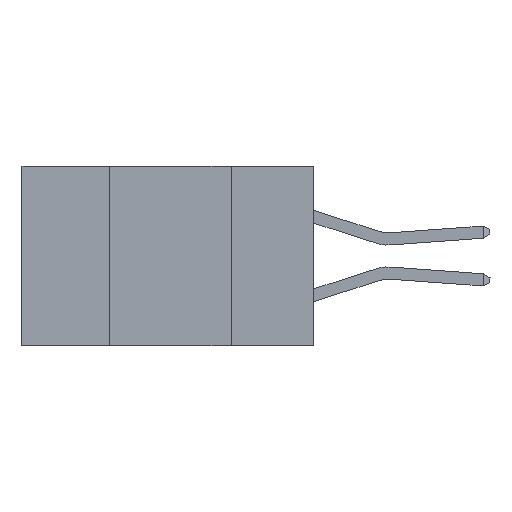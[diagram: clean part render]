
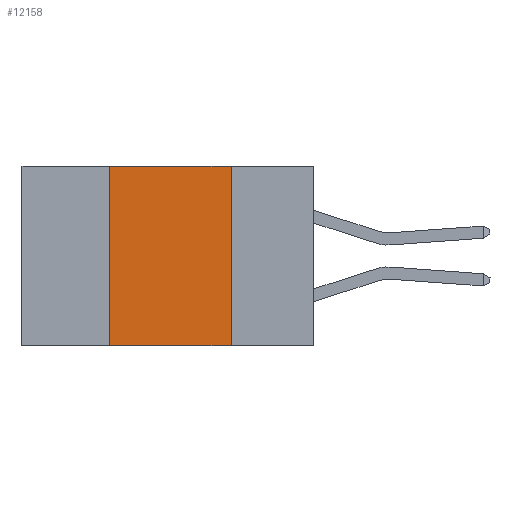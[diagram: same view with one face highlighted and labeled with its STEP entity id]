
A CAD part, left-side view. The second image highlights one B-rep face of the part: STEP entity #12158.
In plain terms, the highlighted planar face has unit normal (-1, 0, 0).
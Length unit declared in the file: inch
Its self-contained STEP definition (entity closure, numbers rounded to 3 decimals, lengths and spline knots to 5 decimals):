
#51 = EDGE_CURVE ( 'NONE', #9231, #17486, #16241, .T. ) ;
#1296 = ORIENTED_EDGE ( 'NONE', *, *, #18186, .F. ) ;
#1807 = VECTOR ( 'NONE', #5083, 39.37008 ) ;
#2206 = CARTESIAN_POINT ( 'NONE',  ( 0., 0.17, 0. ) ) ;
#2783 = DIRECTION ( 'NONE',  ( 0., 0., -1. ) ) ;
#3113 = VECTOR ( 'NONE', #12001, 39.37008 ) ;
#3127 = ORIENTED_EDGE ( 'NONE', *, *, #18317, .F. ) ;
#3414 = CARTESIAN_POINT ( 'NONE',  ( 0., 0.42, 0. ) ) ;
#3640 = LINE ( 'NONE', #10386, #3113 ) ;
#4039 = CARTESIAN_POINT ( 'NONE',  ( 0., 0.6, -0.37 ) ) ;
#5083 = DIRECTION ( 'NONE',  ( 0., 0., 1. ) ) ;
#5323 = EDGE_LOOP ( 'NONE', ( #15356, #3127, #1296, #19670 ) ) ;
#6427 = LINE ( 'NONE', #11020, #19567 ) ;
#7579 = CARTESIAN_POINT ( 'NONE',  ( 0., 0.6, 0. ) ) ;
#8366 = VERTEX_POINT ( 'NONE', #2206 ) ;
#9231 = VERTEX_POINT ( 'NONE', #12782 ) ;
#9264 = DIRECTION ( 'NONE',  ( 0., 0., -1. ) ) ;
#9937 = CARTESIAN_POINT ( 'NONE',  ( 0., 0.17, -0.37 ) ) ;
#10386 = CARTESIAN_POINT ( 'NONE',  ( 0., 0.6, 0. ) ) ;
#10486 = EDGE_CURVE ( 'NONE', #8366, #17486, #6427, .T. ) ;
#10647 = LINE ( 'NONE', #3414, #1807 ) ;
#10839 = VECTOR ( 'NONE', #17237, 39.37008 ) ;
#11020 = CARTESIAN_POINT ( 'NONE',  ( 0., 0.17, 0. ) ) ;
#12001 = DIRECTION ( 'NONE',  ( 0., -1., 0. ) ) ;
#12158 = ADVANCED_FACE ( 'NONE', ( #16659 ), #14101, .F. ) ;
#12782 = CARTESIAN_POINT ( 'NONE',  ( 0., 0.42, -0.37 ) ) ;
#14101 = PLANE ( 'NONE',  #20861 ) ;
#15356 = ORIENTED_EDGE ( 'NONE', *, *, #10486, .F. ) ;
#16241 = LINE ( 'NONE', #4039, #10839 ) ;
#16659 = FACE_OUTER_BOUND ( 'NONE', #5323, .T. ) ;
#17237 = DIRECTION ( 'NONE',  ( 0., -1., 0. ) ) ;
#17374 = CARTESIAN_POINT ( 'NONE',  ( 0., 0.42, 0. ) ) ;
#17486 = VERTEX_POINT ( 'NONE', #9937 ) ;
#18186 = EDGE_CURVE ( 'NONE', #9231, #20870, #10647, .T. ) ;
#18317 = EDGE_CURVE ( 'NONE', #20870, #8366, #3640, .T. ) ;
#19077 = DIRECTION ( 'NONE',  ( 1., 0., 0. ) ) ;
#19567 = VECTOR ( 'NONE', #2783, 39.37008 ) ;
#19670 = ORIENTED_EDGE ( 'NONE', *, *, #51, .T. ) ;
#20861 = AXIS2_PLACEMENT_3D ( 'NONE', #7579, #19077, #9264 ) ;
#20870 = VERTEX_POINT ( 'NONE', #17374 ) ;
